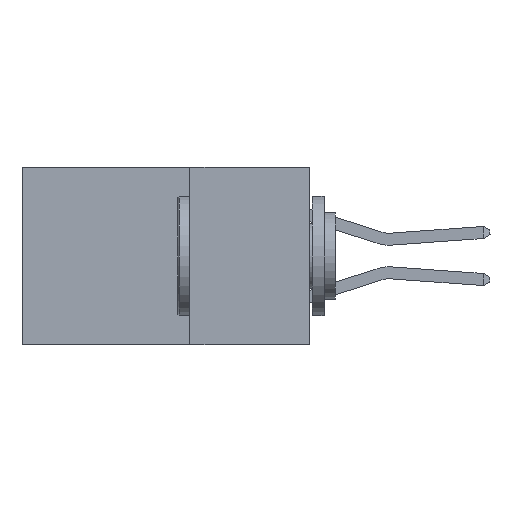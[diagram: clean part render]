
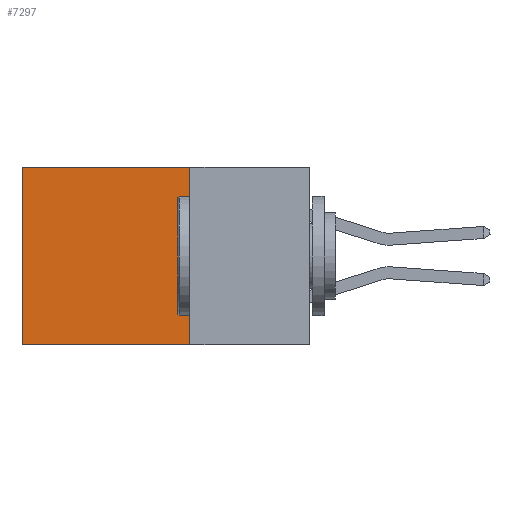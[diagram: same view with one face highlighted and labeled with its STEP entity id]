
A CAD part, left-side view. The second image highlights one B-rep face of the part: STEP entity #7297.
In plain terms, the highlighted planar face has unit normal (-1, 0, 0).
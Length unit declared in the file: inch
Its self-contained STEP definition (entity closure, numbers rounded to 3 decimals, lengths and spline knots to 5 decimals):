
#920 = CARTESIAN_POINT ( 'NONE',  ( 0.2615, 0.25, -0.37 ) ) ;
#1897 = AXIS2_PLACEMENT_3D ( 'NONE', #17705, #25507, #7923 ) ;
#2800 = CARTESIAN_POINT ( 'NONE',  ( 0.2615, 0.25, -0.37 ) ) ;
#4143 = CARTESIAN_POINT ( 'NONE',  ( 0.2615, 0.6, 0. ) ) ;
#4301 = EDGE_CURVE ( 'NONE', #11322, #12255, #18707, .T. ) ;
#4371 = DIRECTION ( 'NONE',  ( 0., 0., -1. ) ) ;
#5049 = VERTEX_POINT ( 'NONE', #4143 ) ;
#5705 = FACE_OUTER_BOUND ( 'NONE', #19439, .T. ) ;
#5894 = EDGE_CURVE ( 'NONE', #11322, #5049, #20006, .T. ) ;
#5990 = CARTESIAN_POINT ( 'NONE',  ( 0.2615, 0.25, 0. ) ) ;
#7297 = ADVANCED_FACE ( 'NONE', ( #5705 ), #9754, .F. ) ;
#7732 = CARTESIAN_POINT ( 'NONE',  ( 0.2615, 0.6, -0.37 ) ) ;
#7923 = DIRECTION ( 'NONE',  ( 0., 0., -1. ) ) ;
#9074 = ORIENTED_EDGE ( 'NONE', *, *, #25347, .T. ) ;
#9754 = PLANE ( 'NONE',  #1897 ) ;
#9829 = DIRECTION ( 'NONE',  ( 0., 1., 0. ) ) ;
#9860 = DIRECTION ( 'NONE',  ( 0., 1., 0. ) ) ;
#10360 = CARTESIAN_POINT ( 'NONE',  ( 0.2615, 0.25, 0. ) ) ;
#10579 = VECTOR ( 'NONE', #4371, 39.37008 ) ;
#11221 = DIRECTION ( 'NONE',  ( 0., 0., -1. ) ) ;
#11322 = VERTEX_POINT ( 'NONE', #5990 ) ;
#11797 = CARTESIAN_POINT ( 'NONE',  ( 0.2615, 0.25, -0.37 ) ) ;
#12255 = VERTEX_POINT ( 'NONE', #920 ) ;
#13210 = ORIENTED_EDGE ( 'NONE', *, *, #4301, .F. ) ;
#13518 = EDGE_CURVE ( 'NONE', #12255, #18770, #20238, .T. ) ;
#13769 = VECTOR ( 'NONE', #9829, 39.37008 ) ;
#14857 = LINE ( 'NONE', #17335, #20541 ) ;
#16467 = ORIENTED_EDGE ( 'NONE', *, *, #13518, .F. ) ;
#17335 = CARTESIAN_POINT ( 'NONE',  ( 0.2615, 0.6, -0.37 ) ) ;
#17705 = CARTESIAN_POINT ( 'NONE',  ( 0.2615, 0.25, -0.37 ) ) ;
#18707 = LINE ( 'NONE', #2800, #10579 ) ;
#18770 = VERTEX_POINT ( 'NONE', #7732 ) ;
#19439 = EDGE_LOOP ( 'NONE', ( #9074, #16467, #13210, #24896 ) ) ;
#20006 = LINE ( 'NONE', #10360, #25147 ) ;
#20238 = LINE ( 'NONE', #11797, #13769 ) ;
#20541 = VECTOR ( 'NONE', #11221, 39.37008 ) ;
#24896 = ORIENTED_EDGE ( 'NONE', *, *, #5894, .T. ) ;
#25147 = VECTOR ( 'NONE', #9860, 39.37008 ) ;
#25347 = EDGE_CURVE ( 'NONE', #5049, #18770, #14857, .T. ) ;
#25507 = DIRECTION ( 'NONE',  ( 1., 0., 0. ) ) ;
